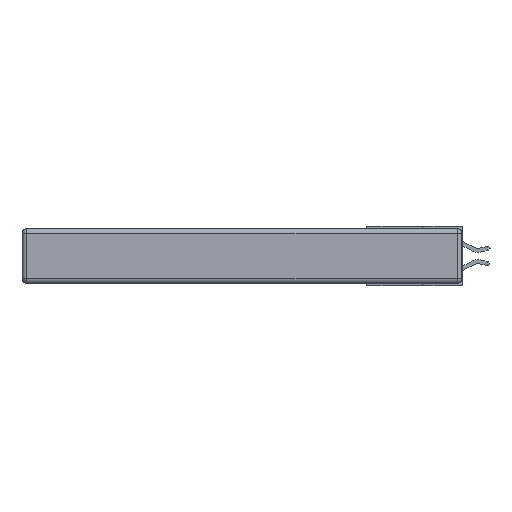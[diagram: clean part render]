
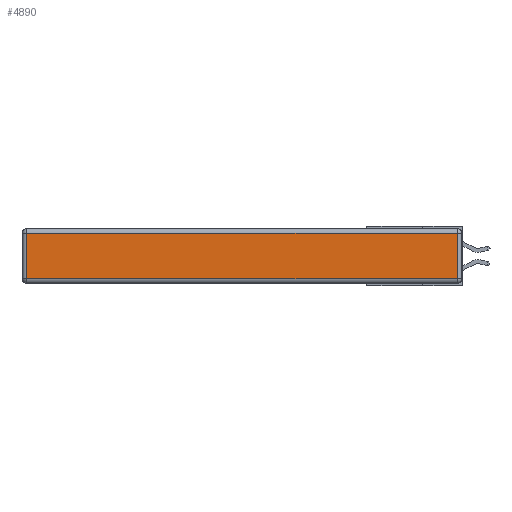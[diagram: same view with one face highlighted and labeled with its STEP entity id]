
A CAD part, left-side view. The second image highlights one B-rep face of the part: STEP entity #4890.
In plain terms, the highlighted planar face has unit normal (-1, 0, 0).
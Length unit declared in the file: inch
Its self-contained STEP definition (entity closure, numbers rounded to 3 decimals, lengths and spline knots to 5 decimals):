
#1026 = DIRECTION ( 'NONE',  ( 0., 0., -1. ) ) ;
#1573 = FACE_OUTER_BOUND ( 'NONE', #24406, .T. ) ;
#1704 = EDGE_CURVE ( 'NONE', #23912, #21066, #23201, .T. ) ;
#3194 = EDGE_CURVE ( 'NONE', #21066, #19023, #6818, .T. ) ;
#3842 = EDGE_CURVE ( 'NONE', #19023, #19730, #8671, .T. ) ;
#4890 = ADVANCED_FACE ( 'NONE', ( #1573 ), #7782, .T. ) ;
#4899 = ORIENTED_EDGE ( 'NONE', *, *, #3194, .T. ) ;
#5028 = CARTESIAN_POINT ( 'NONE',  ( 0., 2.72, -0.343 ) ) ;
#5622 = DIRECTION ( 'NONE',  ( 0., 1., 0. ) ) ;
#5681 = LINE ( 'NONE', #18272, #21397 ) ;
#5716 = ORIENTED_EDGE ( 'NONE', *, *, #16016, .T. ) ;
#6818 = LINE ( 'NONE', #5028, #15445 ) ;
#7160 = CARTESIAN_POINT ( 'NONE',  ( 0., 2.72, -0.03 ) ) ;
#7782 = PLANE ( 'NONE',  #10447 ) ;
#8671 = LINE ( 'NONE', #15492, #17666 ) ;
#10225 = CARTESIAN_POINT ( 'NONE',  ( 0., 2.72, -0.313 ) ) ;
#10447 = AXIS2_PLACEMENT_3D ( 'NONE', #14098, #26088, #21961 ) ;
#10812 = CARTESIAN_POINT ( 'NONE',  ( 0., 0.03, -0.03 ) ) ;
#11700 = VECTOR ( 'NONE', #5622, 39.37008 ) ;
#12044 = ORIENTED_EDGE ( 'NONE', *, *, #3842, .T. ) ;
#14098 = CARTESIAN_POINT ( 'NONE',  ( 0., 0., -0.343 ) ) ;
#15445 = VECTOR ( 'NONE', #1026, 39.37008 ) ;
#15492 = CARTESIAN_POINT ( 'NONE',  ( 0., 0., -0.313 ) ) ;
#16016 = EDGE_CURVE ( 'NONE', #19730, #23912, #5681, .T. ) ;
#17666 = VECTOR ( 'NONE', #25800, 39.37008 ) ;
#17925 = CARTESIAN_POINT ( 'NONE',  ( 0., 2.75, -0.03 ) ) ;
#18272 = CARTESIAN_POINT ( 'NONE',  ( 0., 0.03, -0.343 ) ) ;
#19023 = VERTEX_POINT ( 'NONE', #10225 ) ;
#19730 = VERTEX_POINT ( 'NONE', #25719 ) ;
#20331 = DIRECTION ( 'NONE',  ( 0., 0., 1. ) ) ;
#21066 = VERTEX_POINT ( 'NONE', #7160 ) ;
#21397 = VECTOR ( 'NONE', #20331, 39.37008 ) ;
#21961 = DIRECTION ( 'NONE',  ( 0., 0., 1. ) ) ;
#23201 = LINE ( 'NONE', #17925, #11700 ) ;
#23912 = VERTEX_POINT ( 'NONE', #10812 ) ;
#24406 = EDGE_LOOP ( 'NONE', ( #12044, #5716, #24755, #4899 ) ) ;
#24755 = ORIENTED_EDGE ( 'NONE', *, *, #1704, .T. ) ;
#25719 = CARTESIAN_POINT ( 'NONE',  ( 0., 0.03, -0.313 ) ) ;
#25800 = DIRECTION ( 'NONE',  ( 0., -1., 0. ) ) ;
#26088 = DIRECTION ( 'NONE',  ( -1., 0., 0. ) ) ;
